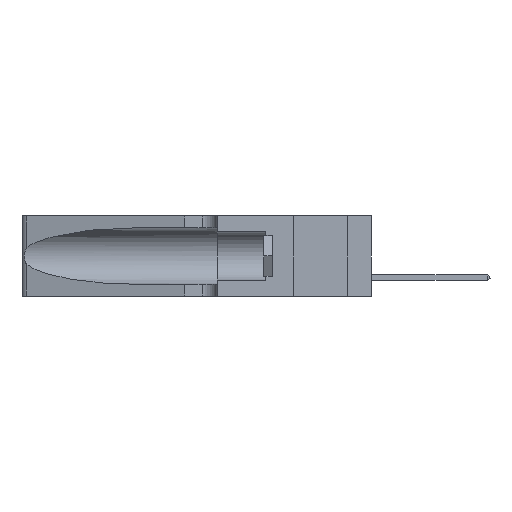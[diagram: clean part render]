
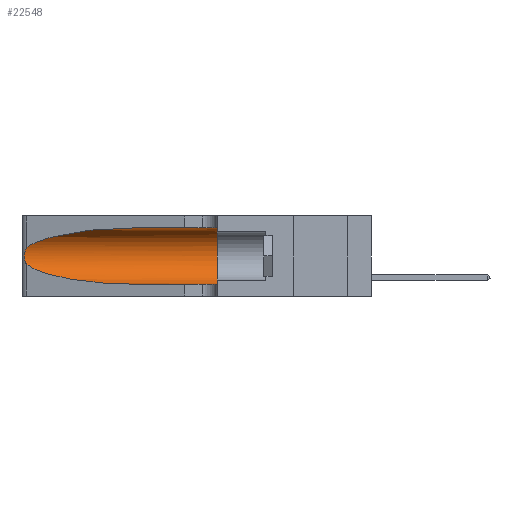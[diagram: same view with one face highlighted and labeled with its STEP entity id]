
A CAD part, left-side view. The second image highlights one B-rep face of the part: STEP entity #22548.
In plain terms, the highlighted cylindrical face has radius 3.308 mm (diameter 6.617 mm), a partial arc.
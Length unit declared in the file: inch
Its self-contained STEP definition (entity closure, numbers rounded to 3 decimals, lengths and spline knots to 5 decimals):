
#1467 = B_SPLINE_CURVE_WITH_KNOTS ( 'NONE', 3,
 ( #37302, #18260, #19984, #23881, #40952, #41136, #28871, #6173, #22012, #36831, #14274, #33486, #29055, #37370 ),
 .UNSPECIFIED., .F., .F.,
 ( 4, 2, 2, 2, 2, 2, 4 ),
 ( 0., 0.00027, 0.00053, 0.00107, 0.0016, 0.00187, 0.00214 ),
 .UNSPECIFIED. ) ;
#1581 = DIRECTION ( 'NONE',  ( 0., 0., 1. ) ) ;
#1654 = VERTEX_POINT ( 'NONE', #8100 ) ;
#2567 = CARTESIAN_POINT ( 'NONE',  ( 0.1305, 0.35, 0.05475 ) ) ;
#3540 = DIRECTION ( 'NONE',  ( 0., -1., 0. ) ) ;
#4132 = ORIENTED_EDGE ( 'NONE', *, *, #27961, .T. ) ;
#4902 = DIRECTION ( 'NONE',  ( 0., -1., 0. ) ) ;
#5322 = DIRECTION ( 'NONE',  ( 0., 1., 0. ) ) ;
#5677 = ORIENTED_EDGE ( 'NONE', *, *, #21427, .T. ) ;
#6173 = CARTESIAN_POINT ( 'NONE',  ( 0.26075, 1.23896, 0.178 ) ) ;
#6829 = DIRECTION ( 'NONE',  ( 0., -1., 0. ) ) ;
#7175 = AXIS2_PLACEMENT_3D ( 'NONE', #17153, #3540, #16674 ) ;
#8100 = CARTESIAN_POINT ( 'NONE',  ( 0.25487, 1.22718, 0.14631 ) ) ;
#8469 = VERTEX_POINT ( 'NONE', #14373 ) ;
#10331 = CARTESIAN_POINT ( 'NONE',  ( 0.1305, 1.61858, 0.31525 ) ) ;
#10498 = CIRCLE ( 'NONE', #34597, 0.13025 ) ;
#10552 = EDGE_LOOP ( 'NONE', ( #30529, #5677, #4132, #45458, #17669, #43386 ) ) ;
#10929 = CARTESIAN_POINT ( 'NONE',  ( 0.1305, 0.72297, 0.05475 ) ) ;
#12161 = CARTESIAN_POINT ( 'NONE',  ( 0.1305, 1.61858, 0.05475 ) ) ;
#12324 = CARTESIAN_POINT ( 'NONE',  ( 0.25487, 1.22718, 0.22369 ) ) ;
#12880 = CARTESIAN_POINT ( 'NONE',  ( 0.1305, 0.72297, 0.31525 ) ) ;
#14150 = CARTESIAN_POINT ( 'NONE',  ( 0.2373, 1.15595, 0.08982 ) ) ;
#14274 = CARTESIAN_POINT ( 'NONE',  ( 0.25789, 1.23486, 0.15765 ) ) ;
#14373 = CARTESIAN_POINT ( 'NONE',  ( 0.1305, 0.72297, 0.31525 ) ) ;
#16272 = CARTESIAN_POINT ( 'NONE',  ( 0.18966, 0.96281, 0.31525 ) ) ;
#16674 = DIRECTION ( 'NONE',  ( 0., 0., -1. ) ) ;
#17153 = CARTESIAN_POINT ( 'NONE',  ( 0.1305, 1.61858, 0.185 ) ) ;
#17638 = CARTESIAN_POINT ( 'NONE',  ( 0.1305, 0.72297, 0.05475 ) ) ;
#17669 = ORIENTED_EDGE ( 'NONE', *, *, #35131, .F. ) ;
#18260 = CARTESIAN_POINT ( 'NONE',  ( 0.25555, 1.22994, 0.2215 ) ) ;
#19030 = LINE ( 'NONE', #12161, #21404 ) ;
#19984 = CARTESIAN_POINT ( 'NONE',  ( 0.25639, 1.23184, 0.21858 ) ) ;
#21404 = VECTOR ( 'NONE', #4902, 39.37008 ) ;
#21427 = EDGE_CURVE ( 'NONE', #25167, #1654, #1467, .T. ) ;
#22012 = CARTESIAN_POINT ( 'NONE',  ( 0.26017, 1.23833, 0.17102 ) ) ;
#22548 = ADVANCED_FACE ( 'NONE', ( #41759 ), #23515, .F. ) ;
#23515 = CYLINDRICAL_SURFACE ( 'NONE', #7175, 0.13025 ) ;
#23881 = CARTESIAN_POINT ( 'NONE',  ( 0.25787, 1.23484, 0.2124 ) ) ;
#25167 = VERTEX_POINT ( 'NONE', #12324 ) ;
#27713 = VERTEX_POINT ( 'NONE', #48674 ) ;
#27961 = EDGE_CURVE ( 'NONE', #1654, #42555, #42117, .T. ) ;
#28871 = CARTESIAN_POINT ( 'NONE',  ( 0.26075, 1.23896, 0.19203 ) ) ;
#29055 = CARTESIAN_POINT ( 'NONE',  ( 0.25555, 1.22993, 0.14849 ) ) ;
#30529 = ORIENTED_EDGE ( 'NONE', *, *, #36906, .T. ) ;
#32610 = CARTESIAN_POINT ( 'NONE',  ( 0.2373, 1.15595, 0.28018 ) ) ;
#33486 = CARTESIAN_POINT ( 'NONE',  ( 0.25639, 1.23186, 0.15144 ) ) ;
#34597 = AXIS2_PLACEMENT_3D ( 'NONE', #47469, #5322, #1581 ) ;
#35131 = EDGE_CURVE ( 'NONE', #27713, #45668, #10498, .T. ) ;
#35708 = EDGE_CURVE ( 'NONE', #8469, #27713, #49735, .T. ) ;
#36831 = CARTESIAN_POINT ( 'NONE',  ( 0.25856, 1.23593, 0.16098 ) ) ;
#36906 = EDGE_CURVE ( 'NONE', #8469, #25167, #47227, .T. ) ;
#37302 = CARTESIAN_POINT ( 'NONE',  ( 0.25487, 1.22718, 0.22369 ) ) ;
#37370 = CARTESIAN_POINT ( 'NONE',  ( 0.25487, 1.22718, 0.14631 ) ) ;
#40952 = CARTESIAN_POINT ( 'NONE',  ( 0.25854, 1.2359, 0.20912 ) ) ;
#41015 = CARTESIAN_POINT ( 'NONE',  ( 0.25487, 1.22718, 0.14631 ) ) ;
#41136 = CARTESIAN_POINT ( 'NONE',  ( 0.26018, 1.23835, 0.19895 ) ) ;
#41759 = FACE_OUTER_BOUND ( 'NONE', #10552, .T. ) ;
#42117 =( BOUNDED_CURVE ( )  B_SPLINE_CURVE ( 3, ( #41015, #14150, #46057, #10929 ),
 .UNSPECIFIED., .F., .T. ) 
 B_SPLINE_CURVE_WITH_KNOTS ( ( 4, 4 ),
 ( 3.44316, 4.71239 ),
 .UNSPECIFIED. ) 
 CURVE ( )  GEOMETRIC_REPRESENTATION_ITEM ( )  RATIONAL_B_SPLINE_CURVE ( ( 1., 0.87, 0.87, 1. ) ) 
 REPRESENTATION_ITEM ( '' )  );
#42555 = VERTEX_POINT ( 'NONE', #17638 ) ;
#43386 = ORIENTED_EDGE ( 'NONE', *, *, #35708, .F. ) ;
#44309 = CARTESIAN_POINT ( 'NONE',  ( 0.25487, 1.22718, 0.22369 ) ) ;
#44847 = VECTOR ( 'NONE', #6829, 39.37008 ) ;
#45458 = ORIENTED_EDGE ( 'NONE', *, *, #49139, .T. ) ;
#45668 = VERTEX_POINT ( 'NONE', #2567 ) ;
#46057 = CARTESIAN_POINT ( 'NONE',  ( 0.18966, 0.96281, 0.05475 ) ) ;
#47227 =( BOUNDED_CURVE ( )  B_SPLINE_CURVE ( 3, ( #12880, #16272, #32610, #44309 ),
 .UNSPECIFIED., .F., .T. ) 
 B_SPLINE_CURVE_WITH_KNOTS ( ( 4, 4 ),
 ( 1.5708, 2.84003 ),
 .UNSPECIFIED. ) 
 CURVE ( )  GEOMETRIC_REPRESENTATION_ITEM ( )  RATIONAL_B_SPLINE_CURVE ( ( 1., 0.87, 0.87, 1. ) ) 
 REPRESENTATION_ITEM ( '' )  );
#47469 = CARTESIAN_POINT ( 'NONE',  ( 0.1305, 0.35, 0.185 ) ) ;
#48674 = CARTESIAN_POINT ( 'NONE',  ( 0.1305, 0.35, 0.31525 ) ) ;
#49139 = EDGE_CURVE ( 'NONE', #42555, #45668, #19030, .T. ) ;
#49735 = LINE ( 'NONE', #10331, #44847 ) ;
